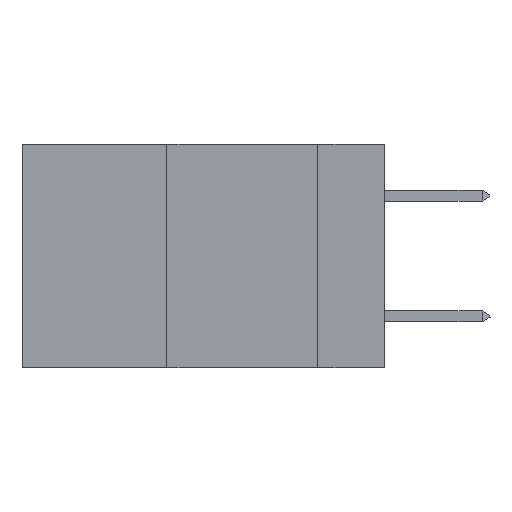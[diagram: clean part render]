
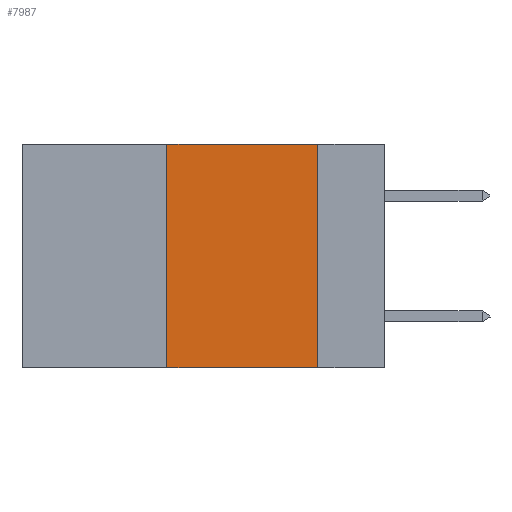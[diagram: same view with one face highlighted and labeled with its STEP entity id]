
A CAD part, left-side view. The second image highlights one B-rep face of the part: STEP entity #7987.
In plain terms, the highlighted planar face has unit normal (-1, 0, 0).
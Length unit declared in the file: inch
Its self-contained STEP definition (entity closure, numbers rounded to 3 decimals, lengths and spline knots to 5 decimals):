
#250 = ORIENTED_EDGE ( 'NONE', *, *, #12272, .F. ) ;
#870 = LINE ( 'NONE', #10860, #23604 ) ;
#882 = ORIENTED_EDGE ( 'NONE', *, *, #3996, .F. ) ;
#1233 = LINE ( 'NONE', #15697, #7640 ) ;
#1273 = ORIENTED_EDGE ( 'NONE', *, *, #22963, .F. ) ;
#3090 = VERTEX_POINT ( 'NONE', #17719 ) ;
#3996 = EDGE_CURVE ( 'NONE', #3090, #18312, #870, .T. ) ;
#5261 = DIRECTION ( 'NONE',  ( 0., 0., 1. ) ) ;
#5458 = DIRECTION ( 'NONE',  ( 0., -1., 0. ) ) ;
#7010 = CARTESIAN_POINT ( 'NONE',  ( 0., 0.11, 0. ) ) ;
#7500 = CARTESIAN_POINT ( 'NONE',  ( 0., 0.6, -0.37 ) ) ;
#7640 = VECTOR ( 'NONE', #15945, 39.37008 ) ;
#7840 = LINE ( 'NONE', #13992, #15155 ) ;
#7987 = ADVANCED_FACE ( 'NONE', ( #16458 ), #16922, .F. ) ;
#8147 = VERTEX_POINT ( 'NONE', #17616 ) ;
#8830 = VERTEX_POINT ( 'NONE', #13490 ) ;
#10698 = DIRECTION ( 'NONE',  ( 0., -1., 0. ) ) ;
#10860 = CARTESIAN_POINT ( 'NONE',  ( 0., 0.6, 0. ) ) ;
#11390 = DIRECTION ( 'NONE',  ( 1., 0., 0. ) ) ;
#11606 = CARTESIAN_POINT ( 'NONE',  ( 0., 0.6, 0. ) ) ;
#12272 = EDGE_CURVE ( 'NONE', #8830, #3090, #7840, .T. ) ;
#13490 = CARTESIAN_POINT ( 'NONE',  ( 0., 0.36, -0.37 ) ) ;
#13864 = AXIS2_PLACEMENT_3D ( 'NONE', #11606, #11390, #23143 ) ;
#13992 = CARTESIAN_POINT ( 'NONE',  ( 0., 0.36, 0. ) ) ;
#14992 = VECTOR ( 'NONE', #5458, 39.37008 ) ;
#15155 = VECTOR ( 'NONE', #5261, 39.37008 ) ;
#15528 = EDGE_CURVE ( 'NONE', #8830, #8147, #22214, .T. ) ;
#15697 = CARTESIAN_POINT ( 'NONE',  ( 0., 0.11, 0. ) ) ;
#15945 = DIRECTION ( 'NONE',  ( 0., 0., -1. ) ) ;
#16263 = EDGE_LOOP ( 'NONE', ( #1273, #882, #250, #18070 ) ) ;
#16458 = FACE_OUTER_BOUND ( 'NONE', #16263, .T. ) ;
#16922 = PLANE ( 'NONE',  #13864 ) ;
#17616 = CARTESIAN_POINT ( 'NONE',  ( 0., 0.11, -0.37 ) ) ;
#17719 = CARTESIAN_POINT ( 'NONE',  ( 0., 0.36, 0. ) ) ;
#18070 = ORIENTED_EDGE ( 'NONE', *, *, #15528, .T. ) ;
#18312 = VERTEX_POINT ( 'NONE', #7010 ) ;
#22214 = LINE ( 'NONE', #7500, #14992 ) ;
#22963 = EDGE_CURVE ( 'NONE', #18312, #8147, #1233, .T. ) ;
#23143 = DIRECTION ( 'NONE',  ( 0., 0., -1. ) ) ;
#23604 = VECTOR ( 'NONE', #10698, 39.37008 ) ;
